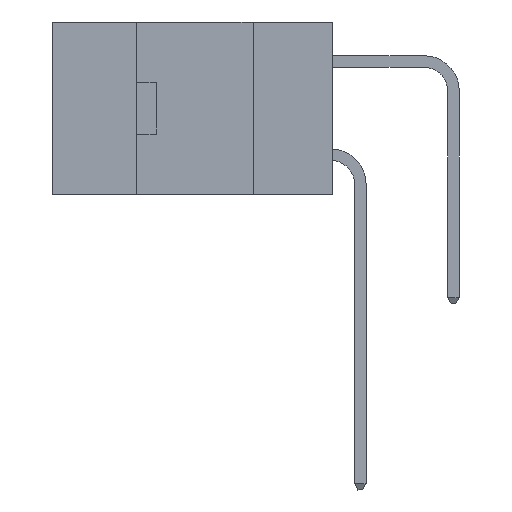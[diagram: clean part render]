
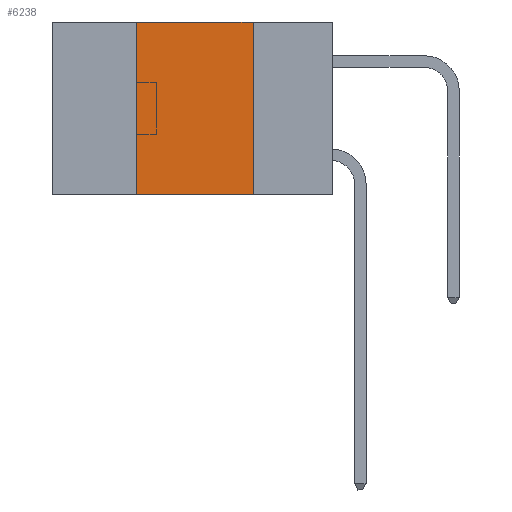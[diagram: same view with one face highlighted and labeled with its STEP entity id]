
A CAD part, left-side view. The second image highlights one B-rep face of the part: STEP entity #6238.
In plain terms, the highlighted planar face has unit normal (-1, 0, 0).
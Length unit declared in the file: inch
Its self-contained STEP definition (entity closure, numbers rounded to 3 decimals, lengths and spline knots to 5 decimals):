
#1038 = DIRECTION ( 'NONE',  ( 0., 0., 1. ) ) ;
#1237 = DIRECTION ( 'NONE',  ( 0., -1., 0. ) ) ;
#1826 = LINE ( 'NONE', #6411, #26330 ) ;
#2168 = PLANE ( 'NONE',  #24747 ) ;
#2447 = CARTESIAN_POINT ( 'NONE',  ( 0., 0.42, -0.37 ) ) ;
#4811 = VECTOR ( 'NONE', #1237, 39.37008 ) ;
#4841 = VERTEX_POINT ( 'NONE', #30328 ) ;
#5124 = VERTEX_POINT ( 'NONE', #10207 ) ;
#6238 = ADVANCED_FACE ( 'NONE', ( #15488 ), #2168, .F. ) ;
#6284 = LINE ( 'NONE', #20396, #4811 ) ;
#6411 = CARTESIAN_POINT ( 'NONE',  ( 0., 0.6, 0. ) ) ;
#9040 = DIRECTION ( 'NONE',  ( 0., -1., 0. ) ) ;
#9418 = DIRECTION ( 'NONE',  ( 1., 0., 0. ) ) ;
#10207 = CARTESIAN_POINT ( 'NONE',  ( 0., 0.17, -0.37 ) ) ;
#12425 = EDGE_CURVE ( 'NONE', #20064, #4841, #15032, .T. ) ;
#13448 = VERTEX_POINT ( 'NONE', #19321 ) ;
#15032 = LINE ( 'NONE', #29407, #26764 ) ;
#15488 = FACE_OUTER_BOUND ( 'NONE', #26967, .T. ) ;
#16862 = ORIENTED_EDGE ( 'NONE', *, *, #20215, .F. ) ;
#17159 = ORIENTED_EDGE ( 'NONE', *, *, #23884, .F. ) ;
#17352 = ORIENTED_EDGE ( 'NONE', *, *, #12425, .F. ) ;
#17492 = CARTESIAN_POINT ( 'NONE',  ( 0., 0.17, -0.37 ) ) ;
#17750 = ORIENTED_EDGE ( 'NONE', *, *, #25829, .T. ) ;
#17921 = VECTOR ( 'NONE', #19880, 39.37008 ) ;
#19321 = CARTESIAN_POINT ( 'NONE',  ( 0., 0.17, 0. ) ) ;
#19405 = LINE ( 'NONE', #17492, #17921 ) ;
#19880 = DIRECTION ( 'NONE',  ( 0., 0., -1. ) ) ;
#20064 = VERTEX_POINT ( 'NONE', #2447 ) ;
#20215 = EDGE_CURVE ( 'NONE', #13448, #5124, #19405, .T. ) ;
#20396 = CARTESIAN_POINT ( 'NONE',  ( 0., 0.6, -0.37 ) ) ;
#23569 = CARTESIAN_POINT ( 'NONE',  ( 0., 0.6, 0. ) ) ;
#23884 = EDGE_CURVE ( 'NONE', #4841, #13448, #1826, .T. ) ;
#24747 = AXIS2_PLACEMENT_3D ( 'NONE', #23569, #9418, #25936 ) ;
#25829 = EDGE_CURVE ( 'NONE', #20064, #5124, #6284, .T. ) ;
#25936 = DIRECTION ( 'NONE',  ( 0., 0., -1. ) ) ;
#26330 = VECTOR ( 'NONE', #9040, 39.37008 ) ;
#26764 = VECTOR ( 'NONE', #1038, 39.37008 ) ;
#26967 = EDGE_LOOP ( 'NONE', ( #16862, #17159, #17352, #17750 ) ) ;
#29407 = CARTESIAN_POINT ( 'NONE',  ( 0., 0.42, -0.37 ) ) ;
#30328 = CARTESIAN_POINT ( 'NONE',  ( 0., 0.42, 0. ) ) ;
